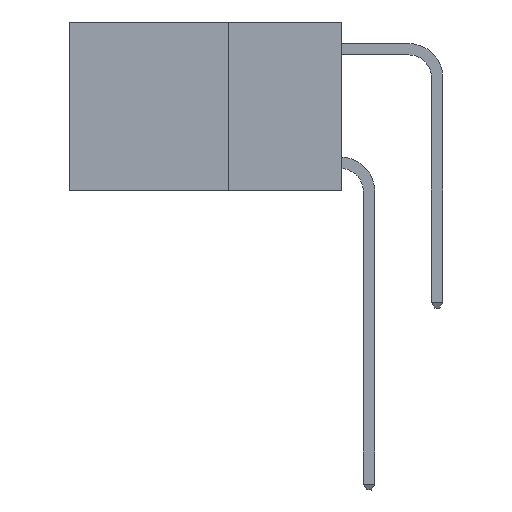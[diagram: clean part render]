
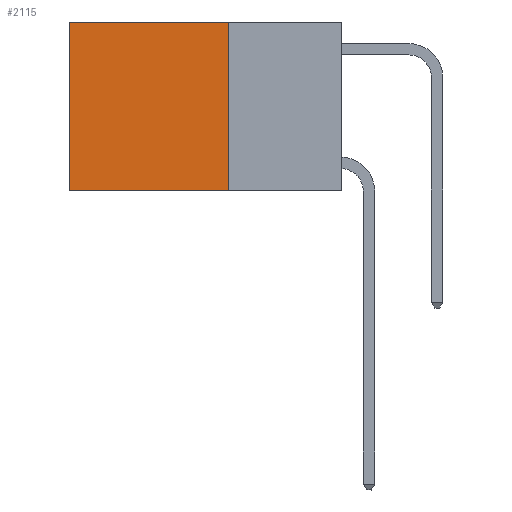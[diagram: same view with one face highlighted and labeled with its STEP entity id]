
A CAD part, left-side view. The second image highlights one B-rep face of the part: STEP entity #2115.
In plain terms, the highlighted planar face has unit normal (-1, 0, 0).
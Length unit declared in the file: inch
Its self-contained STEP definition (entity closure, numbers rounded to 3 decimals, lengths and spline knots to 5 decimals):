
#183 = LINE ( 'NONE', #1741, #7710 ) ;
#1232 = PLANE ( 'NONE',  #3021 ) ;
#1741 = CARTESIAN_POINT ( 'NONE',  ( 0.2625, 0.25, 0. ) ) ;
#1988 = VERTEX_POINT ( 'NONE', #9862 ) ;
#2115 = ADVANCED_FACE ( 'NONE', ( #10193 ), #1232, .F. ) ;
#2213 = VECTOR ( 'NONE', #10537, 39.37008 ) ;
#2242 = VECTOR ( 'NONE', #8686, 39.37008 ) ;
#2250 = ORIENTED_EDGE ( 'NONE', *, *, #14590, .F. ) ;
#2272 = CARTESIAN_POINT ( 'NONE',  ( 0.2625, 0.6, 0. ) ) ;
#2499 = EDGE_LOOP ( 'NONE', ( #5653, #2250, #12744, #9180 ) ) ;
#3021 = AXIS2_PLACEMENT_3D ( 'NONE', #10265, #4855, #12746 ) ;
#3174 = EDGE_CURVE ( 'NONE', #11358, #14299, #12331, .T. ) ;
#3639 = CARTESIAN_POINT ( 'NONE',  ( 0.2625, 0.25, 0. ) ) ;
#4855 = DIRECTION ( 'NONE',  ( 1., 0., 0. ) ) ;
#5653 = ORIENTED_EDGE ( 'NONE', *, *, #3174, .T. ) ;
#7142 = VECTOR ( 'NONE', #13031, 39.37008 ) ;
#7710 = VECTOR ( 'NONE', #13201, 39.37008 ) ;
#8190 = EDGE_CURVE ( 'NONE', #14679, #1988, #183, .T. ) ;
#8686 = DIRECTION ( 'NONE',  ( 0., 0., -1. ) ) ;
#9180 = ORIENTED_EDGE ( 'NONE', *, *, #11888, .T. ) ;
#9862 = CARTESIAN_POINT ( 'NONE',  ( 0.2625, 0.25, -0.37 ) ) ;
#10193 = FACE_OUTER_BOUND ( 'NONE', #2499, .T. ) ;
#10265 = CARTESIAN_POINT ( 'NONE',  ( 0.2625, 0.25, 0. ) ) ;
#10537 = DIRECTION ( 'NONE',  ( 0., 1., 0. ) ) ;
#11224 = CARTESIAN_POINT ( 'NONE',  ( 0.2625, 0.6, -0.37 ) ) ;
#11358 = VERTEX_POINT ( 'NONE', #2272 ) ;
#11874 = CARTESIAN_POINT ( 'NONE',  ( 0.2625, 0.25, -0.37 ) ) ;
#11888 = EDGE_CURVE ( 'NONE', #14679, #11358, #11924, .T. ) ;
#11924 = LINE ( 'NONE', #3639, #2213 ) ;
#12012 = LINE ( 'NONE', #11874, #7142 ) ;
#12331 = LINE ( 'NONE', #14513, #2242 ) ;
#12744 = ORIENTED_EDGE ( 'NONE', *, *, #8190, .F. ) ;
#12746 = DIRECTION ( 'NONE',  ( 0., 0., -1. ) ) ;
#13031 = DIRECTION ( 'NONE',  ( 0., 1., 0. ) ) ;
#13201 = DIRECTION ( 'NONE',  ( 0., 0., -1. ) ) ;
#14299 = VERTEX_POINT ( 'NONE', #11224 ) ;
#14354 = CARTESIAN_POINT ( 'NONE',  ( 0.2625, 0.25, 0. ) ) ;
#14513 = CARTESIAN_POINT ( 'NONE',  ( 0.2625, 0.6, 0. ) ) ;
#14590 = EDGE_CURVE ( 'NONE', #1988, #14299, #12012, .T. ) ;
#14679 = VERTEX_POINT ( 'NONE', #14354 ) ;
